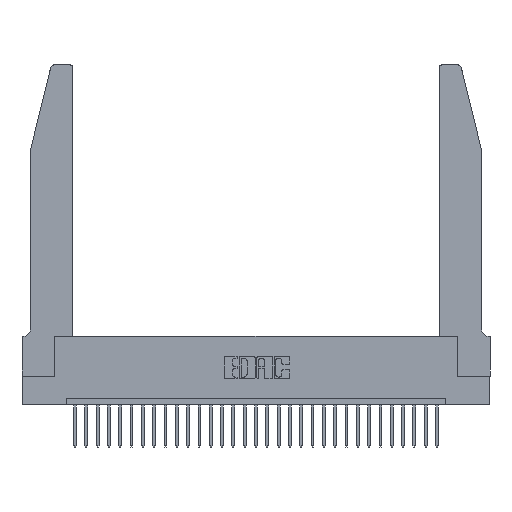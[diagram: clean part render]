
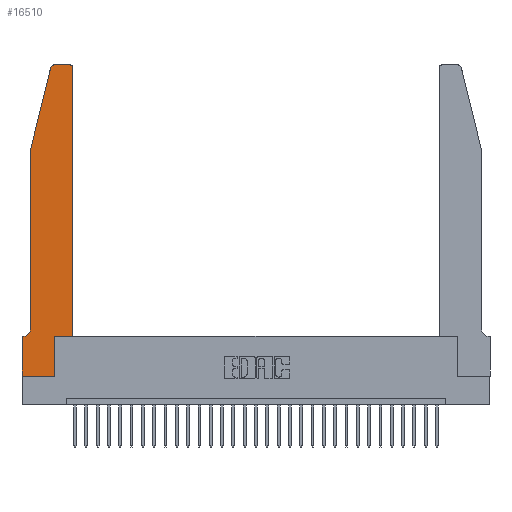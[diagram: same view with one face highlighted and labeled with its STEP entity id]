
A CAD part, top view. The second image highlights one B-rep face of the part: STEP entity #16510.
In plain terms, the highlighted planar face has unit normal (0, 0, 1).
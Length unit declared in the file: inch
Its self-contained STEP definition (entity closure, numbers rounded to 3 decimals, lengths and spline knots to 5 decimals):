
#311 = AXIS2_PLACEMENT_3D ( 'NONE', #10155, #22369, #12885 ) ;
#655 = DIRECTION ( 'NONE',  ( 0., -1., 0. ) ) ;
#781 = DIRECTION ( 'NONE',  ( -1., 0., 0. ) ) ;
#1009 = LINE ( 'NONE', #10876, #15529 ) ;
#2777 = LINE ( 'NONE', #14198, #19907 ) ;
#2864 = VERTEX_POINT ( 'NONE', #3496 ) ;
#3156 = ORIENTED_EDGE ( 'NONE', *, *, #15985, .T. ) ;
#3208 = EDGE_CURVE ( 'NONE', #17580, #12364, #8773, .T. ) ;
#3496 = CARTESIAN_POINT ( 'NONE',  ( 0., 0.35, 0.37 ) ) ;
#3731 = DIRECTION ( 'NONE',  ( 0., 1., 0. ) ) ;
#4055 = ORIENTED_EDGE ( 'NONE', *, *, #17660, .T. ) ;
#4549 = DIRECTION ( 'NONE',  ( 1., 0., 0. ) ) ;
#5179 = VECTOR ( 'NONE', #3731, 39.37008 ) ;
#5190 = LINE ( 'NONE', #26308, #29739 ) ;
#5795 = DIRECTION ( 'NONE',  ( 1., 0., 0. ) ) ;
#6697 = ORIENTED_EDGE ( 'NONE', *, *, #9988, .T. ) ;
#7038 = LINE ( 'NONE', #24635, #5179 ) ;
#7520 = ORIENTED_EDGE ( 'NONE', *, *, #26832, .T. ) ;
#7628 = CARTESIAN_POINT ( 'NONE',  ( 0.0755, 0.35, 0.37 ) ) ;
#7732 = LINE ( 'NONE', #26446, #12567 ) ;
#7918 = CIRCLE ( 'NONE', #28088, 0.03 ) ;
#7981 = CARTESIAN_POINT ( 'NONE',  ( 0., 0., 0.37 ) ) ;
#8159 = VERTEX_POINT ( 'NONE', #28945 ) ;
#8773 = LINE ( 'NONE', #30741, #11016 ) ;
#8828 = EDGE_CURVE ( 'NONE', #8159, #30793, #1009, .T. ) ;
#9006 = VECTOR ( 'NONE', #781, 39.37008 ) ;
#9109 = ORIENTED_EDGE ( 'NONE', *, *, #19633, .T. ) ;
#9245 = CARTESIAN_POINT ( 'NONE',  ( 0.0755, 0.42, 0.37 ) ) ;
#9254 = CARTESIAN_POINT ( 'NONE',  ( 0.0755, 2., 0.37 ) ) ;
#9988 = EDGE_CURVE ( 'NONE', #15910, #24854, #27380, .T. ) ;
#10155 = CARTESIAN_POINT ( 'NONE',  ( 0.284, 2.72, 0.37 ) ) ;
#10866 = EDGE_CURVE ( 'NONE', #30793, #16915, #20979, .T. ) ;
#10876 = CARTESIAN_POINT ( 'NONE',  ( 0.0755, 2., 0.37 ) ) ;
#11016 = VECTOR ( 'NONE', #25865, 39.37008 ) ;
#11589 = DIRECTION ( 'NONE',  ( -1., 0., 0. ) ) ;
#11653 = DIRECTION ( 'NONE',  ( -0.239, -0.971, 0. ) ) ;
#12161 = VECTOR ( 'NONE', #4549, 39.37008 ) ;
#12364 = VERTEX_POINT ( 'NONE', #24265 ) ;
#12567 = VECTOR ( 'NONE', #655, 39.37008 ) ;
#12885 = DIRECTION ( 'NONE',  ( 1., 0., 0. ) ) ;
#13668 = LINE ( 'NONE', #7981, #12161 ) ;
#13670 = ORIENTED_EDGE ( 'NONE', *, *, #15206, .T. ) ;
#14198 = CARTESIAN_POINT ( 'NONE',  ( 0.4505, 0.35, 0.37 ) ) ;
#14390 = FACE_OUTER_BOUND ( 'NONE', #29678, .T. ) ;
#14804 = VECTOR ( 'NONE', #11653, 39.37008 ) ;
#14842 = ORIENTED_EDGE ( 'NONE', *, *, #25494, .T. ) ;
#15206 = EDGE_CURVE ( 'NONE', #16813, #19887, #7038, .T. ) ;
#15529 = VECTOR ( 'NONE', #15816, 39.37008 ) ;
#15550 = CARTESIAN_POINT ( 'NONE',  ( 0.4205, 2.72, 0.37 ) ) ;
#15816 = DIRECTION ( 'NONE',  ( 0., -1., 0. ) ) ;
#15910 = VERTEX_POINT ( 'NONE', #21158 ) ;
#15985 = EDGE_CURVE ( 'NONE', #24854, #8159, #25225, .T. ) ;
#16231 = DIRECTION ( 'NONE',  ( 0., 0., -1. ) ) ;
#16431 = EDGE_CURVE ( 'NONE', #25742, #16813, #13668, .T. ) ;
#16510 = ADVANCED_FACE ( 'NONE', ( #14390 ), #29221, .T. ) ;
#16813 = VERTEX_POINT ( 'NONE', #22370 ) ;
#16915 = VERTEX_POINT ( 'NONE', #21477 ) ;
#17580 = VERTEX_POINT ( 'NONE', #25619 ) ;
#17660 = EDGE_CURVE ( 'NONE', #19887, #17580, #2777, .T. ) ;
#17973 = CARTESIAN_POINT ( 'NONE',  ( 0.4205, 2.75, 0.37 ) ) ;
#19162 = ORIENTED_EDGE ( 'NONE', *, *, #22994, .T. ) ;
#19394 = CARTESIAN_POINT ( 'NONE',  ( 0.25487, 2.72718, 0.37 ) ) ;
#19633 = EDGE_CURVE ( 'NONE', #12364, #24513, #7918, .T. ) ;
#19796 = ORIENTED_EDGE ( 'NONE', *, *, #3208, .T. ) ;
#19887 = VERTEX_POINT ( 'NONE', #23131 ) ;
#19907 = VECTOR ( 'NONE', #21282, 39.37008 ) ;
#20208 = LINE ( 'NONE', #7628, #9006 ) ;
#20938 = ORIENTED_EDGE ( 'NONE', *, *, #16431, .T. ) ;
#20979 = CIRCLE ( 'NONE', #25055, 0.07 ) ;
#21158 = CARTESIAN_POINT ( 'NONE',  ( 0.284, 2.75, 0.37 ) ) ;
#21282 = DIRECTION ( 'NONE',  ( 1., 0., 0. ) ) ;
#21477 = CARTESIAN_POINT ( 'NONE',  ( 0.0055, 0.35, 0.37 ) ) ;
#22369 = DIRECTION ( 'NONE',  ( 0., 0., 1. ) ) ;
#22370 = CARTESIAN_POINT ( 'NONE',  ( 0.2865, 0., 0.37 ) ) ;
#22994 = EDGE_CURVE ( 'NONE', #16915, #2864, #20208, .T. ) ;
#23131 = CARTESIAN_POINT ( 'NONE',  ( 0.2865, 0.35, 0.37 ) ) ;
#24265 = CARTESIAN_POINT ( 'NONE',  ( 0.4505, 2.72, 0.37 ) ) ;
#24513 = VERTEX_POINT ( 'NONE', #17973 ) ;
#24635 = CARTESIAN_POINT ( 'NONE',  ( 0.2865, 0.35, 0.37 ) ) ;
#24835 = CARTESIAN_POINT ( 'NONE',  ( 0., 0.35, 0.37 ) ) ;
#24854 = VERTEX_POINT ( 'NONE', #19394 ) ;
#25055 = AXIS2_PLACEMENT_3D ( 'NONE', #30441, #16231, #11589 ) ;
#25103 = DIRECTION ( 'NONE',  ( 0., 0., 1. ) ) ;
#25145 = ORIENTED_EDGE ( 'NONE', *, *, #10866, .T. ) ;
#25225 = LINE ( 'NONE', #9254, #14804 ) ;
#25494 = EDGE_CURVE ( 'NONE', #2864, #25742, #7732, .T. ) ;
#25619 = CARTESIAN_POINT ( 'NONE',  ( 0.4505, 0.35, 0.37 ) ) ;
#25742 = VERTEX_POINT ( 'NONE', #29453 ) ;
#25865 = DIRECTION ( 'NONE',  ( 0., 1., 0. ) ) ;
#26308 = CARTESIAN_POINT ( 'NONE',  ( 0.2605, 2.75, 0.37 ) ) ;
#26446 = CARTESIAN_POINT ( 'NONE',  ( 0., 0., 0.37 ) ) ;
#26737 = ORIENTED_EDGE ( 'NONE', *, *, #8828, .T. ) ;
#26832 = EDGE_CURVE ( 'NONE', #24513, #15910, #5190, .T. ) ;
#27380 = CIRCLE ( 'NONE', #311, 0.03 ) ;
#28088 = AXIS2_PLACEMENT_3D ( 'NONE', #15550, #25103, #29781 ) ;
#28636 = AXIS2_PLACEMENT_3D ( 'NONE', #24835, #29316, #5795 ) ;
#28803 = DIRECTION ( 'NONE',  ( -1., 0., 0. ) ) ;
#28945 = CARTESIAN_POINT ( 'NONE',  ( 0.0755, 2., 0.37 ) ) ;
#29221 = PLANE ( 'NONE',  #28636 ) ;
#29316 = DIRECTION ( 'NONE',  ( 0., 0., 1. ) ) ;
#29453 = CARTESIAN_POINT ( 'NONE',  ( 0., 0., 0.37 ) ) ;
#29678 = EDGE_LOOP ( 'NONE', ( #7520, #6697, #3156, #26737, #25145, #19162, #14842, #20938, #13670, #4055, #19796, #9109 ) ) ;
#29739 = VECTOR ( 'NONE', #28803, 39.37008 ) ;
#29781 = DIRECTION ( 'NONE',  ( 1., 0., 0. ) ) ;
#30441 = CARTESIAN_POINT ( 'NONE',  ( 0.0055, 0.42, 0.37 ) ) ;
#30741 = CARTESIAN_POINT ( 'NONE',  ( 0.4505, 0.35, 0.37 ) ) ;
#30793 = VERTEX_POINT ( 'NONE', #9245 ) ;
